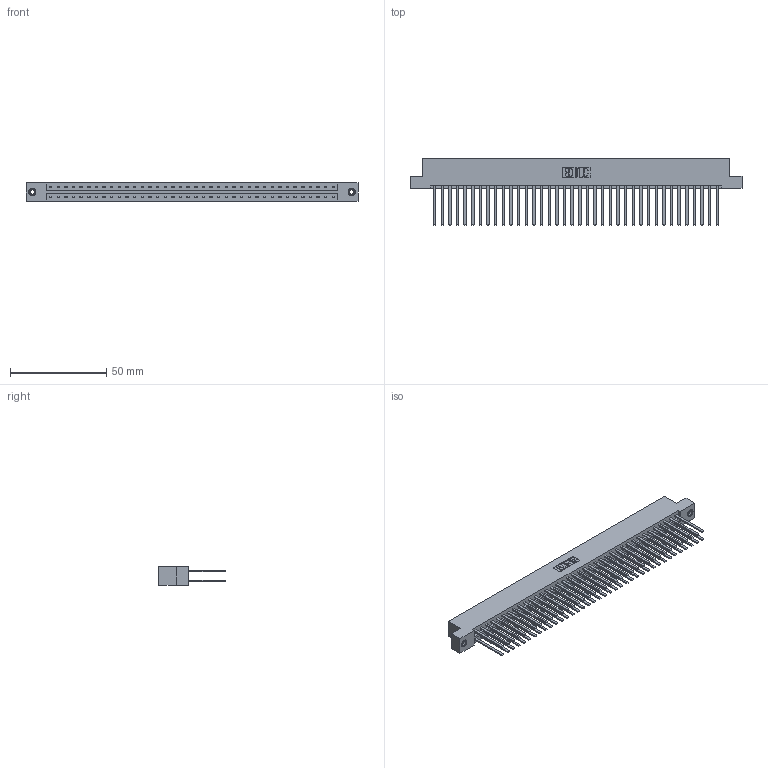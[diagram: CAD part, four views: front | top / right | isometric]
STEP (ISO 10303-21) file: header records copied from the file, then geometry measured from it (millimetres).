
FILE_DESCRIPTION (( 'STEP AP203' ), '1' );
FILE_NAME ('333-076-544-208.STEP', '2018-08-04T23:15:22', ( '' ), ( '' ), 'SwSTEP 2.0', 'SolidWorks 2016', '' );
FILE_SCHEMA (( 'CONFIG_CONTROL_DESIGN' ));
Length unit declared in the file: inch
Products named in the file (4): 333 Part_Flush - .156 Dia - TI; 345-292-001_345-293-144; 345-250-001_345-250-003-102; 333-076-544-208
Assembly tree (79 placements, depth 2):
  333-076-544-208
    333 Part_Flush - .156 Dia - TI
    345-292-001_345-293-144  x76
    345-250-001_345-250-003-102  x2
Bounding box: 172.11 x 34.3 x 9.4 mm (x, y, z)
Volume: 18592.9 mm3; surface area: 25390.5 mm2
Topology: 79 solids, 79 shells, 3670 faces, 10859 edges, 7130 vertices
Faces by surface type: plane 2534, cylinder 1120, cone 12, torus 4
Entity records: 25966 total; most frequent: CARTESIAN_POINT 4289, ORIENTED_EDGE 4218, DIRECTION 3699, EDGE_CURVE 2109, VECTOR 1965, LINE 1965, VERTEX_POINT 1400, AXIS2_PLACEMENT_3D 867
